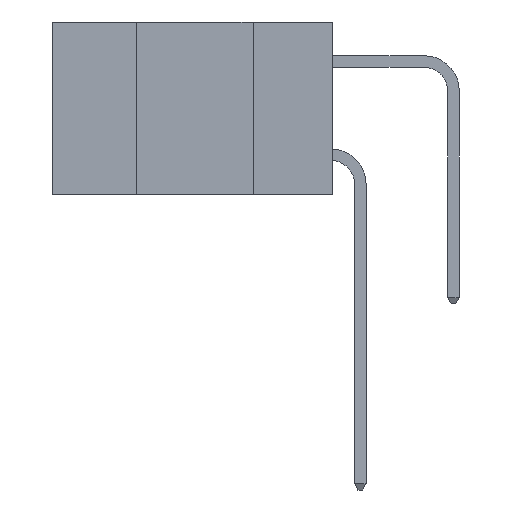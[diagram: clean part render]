
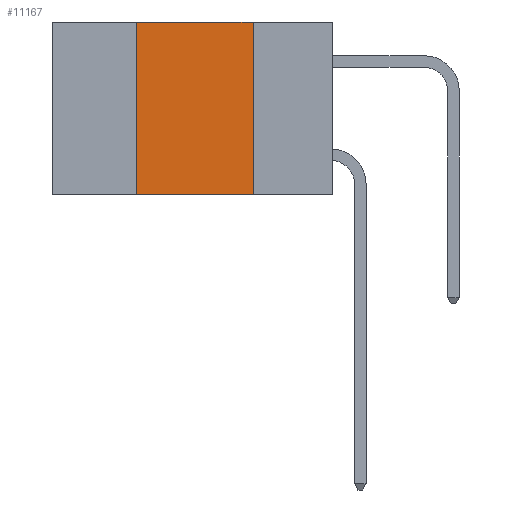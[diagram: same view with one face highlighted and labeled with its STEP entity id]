
A CAD part, left-side view. The second image highlights one B-rep face of the part: STEP entity #11167.
In plain terms, the highlighted planar face has unit normal (-1, 0, 0).
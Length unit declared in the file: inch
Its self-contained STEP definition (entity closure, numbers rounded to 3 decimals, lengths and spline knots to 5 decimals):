
#637 = ORIENTED_EDGE ( 'NONE', *, *, #18541, .F. ) ;
#1933 = ORIENTED_EDGE ( 'NONE', *, *, #4300, .F. ) ;
#2036 = EDGE_LOOP ( 'NONE', ( #637, #11397, #1933, #13258 ) ) ;
#2603 = LINE ( 'NONE', #13193, #7972 ) ;
#3491 = VECTOR ( 'NONE', #15502, 39.37008 ) ;
#4300 = EDGE_CURVE ( 'NONE', #19895, #9584, #22782, .T. ) ;
#4643 = PLANE ( 'NONE',  #9266 ) ;
#4906 = CARTESIAN_POINT ( 'NONE',  ( 0., 0.42, -0.37 ) ) ;
#6653 = DIRECTION ( 'NONE',  ( 1., 0., 0. ) ) ;
#6874 = VECTOR ( 'NONE', #8925, 39.37008 ) ;
#7014 = EDGE_CURVE ( 'NONE', #9584, #17043, #2603, .T. ) ;
#7972 = VECTOR ( 'NONE', #19185, 39.37008 ) ;
#8925 = DIRECTION ( 'NONE',  ( 0., 0., 1. ) ) ;
#9266 = AXIS2_PLACEMENT_3D ( 'NONE', #18601, #6653, #20616 ) ;
#9584 = VERTEX_POINT ( 'NONE', #22694 ) ;
#10055 = VECTOR ( 'NONE', #24818, 39.37008 ) ;
#11167 = ADVANCED_FACE ( 'NONE', ( #13764 ), #4643, .F. ) ;
#11397 = ORIENTED_EDGE ( 'NONE', *, *, #7014, .F. ) ;
#12014 = CARTESIAN_POINT ( 'NONE',  ( 0., 0.17, -0.37 ) ) ;
#13193 = CARTESIAN_POINT ( 'NONE',  ( 0., 0.6, 0. ) ) ;
#13258 = ORIENTED_EDGE ( 'NONE', *, *, #25709, .T. ) ;
#13611 = CARTESIAN_POINT ( 'NONE',  ( 0., 0.42, -0.37 ) ) ;
#13764 = FACE_OUTER_BOUND ( 'NONE', #2036, .T. ) ;
#15502 = DIRECTION ( 'NONE',  ( 0., -1., 0. ) ) ;
#17043 = VERTEX_POINT ( 'NONE', #20597 ) ;
#18192 = VERTEX_POINT ( 'NONE', #12014 ) ;
#18541 = EDGE_CURVE ( 'NONE', #17043, #18192, #20664, .T. ) ;
#18601 = CARTESIAN_POINT ( 'NONE',  ( 0., 0.6, 0. ) ) ;
#19185 = DIRECTION ( 'NONE',  ( 0., -1., 0. ) ) ;
#19417 = CARTESIAN_POINT ( 'NONE',  ( 0., 0.6, -0.37 ) ) ;
#19895 = VERTEX_POINT ( 'NONE', #13611 ) ;
#20597 = CARTESIAN_POINT ( 'NONE',  ( 0., 0.17, 0. ) ) ;
#20616 = DIRECTION ( 'NONE',  ( 0., 0., -1. ) ) ;
#20664 = LINE ( 'NONE', #20871, #10055 ) ;
#20871 = CARTESIAN_POINT ( 'NONE',  ( 0., 0.17, -0.37 ) ) ;
#22694 = CARTESIAN_POINT ( 'NONE',  ( 0., 0.42, 0. ) ) ;
#22782 = LINE ( 'NONE', #4906, #6874 ) ;
#24676 = LINE ( 'NONE', #19417, #3491 ) ;
#24818 = DIRECTION ( 'NONE',  ( 0., 0., -1. ) ) ;
#25709 = EDGE_CURVE ( 'NONE', #19895, #18192, #24676, .T. ) ;
